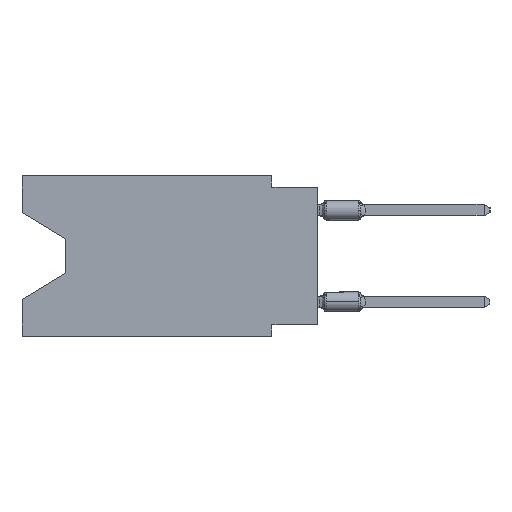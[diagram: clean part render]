
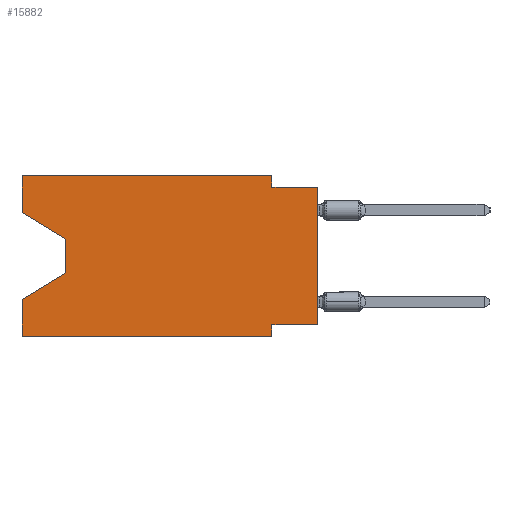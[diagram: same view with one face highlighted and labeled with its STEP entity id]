
A CAD part, left-side view. The second image highlights one B-rep face of the part: STEP entity #15882.
In plain terms, the highlighted planar face has unit normal (-1, 0, 0).
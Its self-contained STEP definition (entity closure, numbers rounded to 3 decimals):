
#258 = VERTEX_POINT ( 'NONE', #11787 ) ;
#295 = CARTESIAN_POINT ( 'NONE',  ( 0., 16.383, 0. ) ) ;
#421 = ORIENTED_EDGE ( 'NONE', *, *, #10246, .F. ) ;
#449 = DIRECTION ( 'NONE',  ( 0., 0., 1. ) ) ;
#477 = VECTOR ( 'NONE', #29039, 1000. ) ;
#811 = VERTEX_POINT ( 'NONE', #11606 ) ;
#919 = VERTEX_POINT ( 'NONE', #9979 ) ;
#1037 = CARTESIAN_POINT ( 'NONE',  ( 0., 13.97, -3.505 ) ) ;
#1049 = VECTOR ( 'NONE', #26966, 1000. ) ;
#1107 = DIRECTION ( 'NONE',  ( 0., 1., 0. ) ) ;
#1323 = VERTEX_POINT ( 'NONE', #10096 ) ;
#1405 = CARTESIAN_POINT ( 'NONE',  ( 0., 16.383, -2.038 ) ) ;
#1774 = LINE ( 'NONE', #10872, #17220 ) ;
#1942 = LINE ( 'NONE', #20669, #10869 ) ;
#2141 = DIRECTION ( 'NONE',  ( 0., 0., -1. ) ) ;
#2292 = LINE ( 'NONE', #16287, #26268 ) ;
#2627 = ORIENTED_EDGE ( 'NONE', *, *, #11034, .F. ) ;
#3143 = DIRECTION ( 'NONE',  ( 0., 0., -1. ) ) ;
#3169 = CARTESIAN_POINT ( 'NONE',  ( 0., 16.383, 0. ) ) ;
#3253 = EDGE_CURVE ( 'NONE', #1323, #10545, #4941, .T. ) ;
#3548 = VERTEX_POINT ( 'NONE', #3169 ) ;
#3642 = CARTESIAN_POINT ( 'NONE',  ( 0., 16.383, -6.852 ) ) ;
#3846 = AXIS2_PLACEMENT_3D ( 'NONE', #5062, #14456, #3143 ) ;
#3945 = VERTEX_POINT ( 'NONE', #5924 ) ;
#4104 = EDGE_CURVE ( 'NONE', #21674, #27669, #26607, .T. ) ;
#4353 = CARTESIAN_POINT ( 'NONE',  ( 0., 2.54, -0.635 ) ) ;
#4443 = DIRECTION ( 'NONE',  ( 0., 0., -1. ) ) ;
#4531 = LINE ( 'NONE', #22835, #7542 ) ;
#4649 = DIRECTION ( 'NONE',  ( 0., 0., 1. ) ) ;
#4802 = CARTESIAN_POINT ( 'NONE',  ( 0., 0., 0. ) ) ;
#4941 = LINE ( 'NONE', #4802, #22387 ) ;
#5062 = CARTESIAN_POINT ( 'NONE',  ( 0., 16.383, 0. ) ) ;
#5570 = CARTESIAN_POINT ( 'NONE',  ( 0., 0., -8.255 ) ) ;
#5795 = ORIENTED_EDGE ( 'NONE', *, *, #9976, .F. ) ;
#5924 = CARTESIAN_POINT ( 'NONE',  ( 0., 2.54, 0. ) ) ;
#6217 = DIRECTION ( 'NONE',  ( 0., 0.855, -0.519 ) ) ;
#6565 = ORIENTED_EDGE ( 'NONE', *, *, #16630, .F. ) ;
#7277 = EDGE_CURVE ( 'NONE', #25201, #27669, #26378, .T. ) ;
#7542 = VECTOR ( 'NONE', #9296, 1000. ) ;
#7638 = EDGE_CURVE ( 'NONE', #258, #21674, #21414, .T. ) ;
#7674 = CARTESIAN_POINT ( 'NONE',  ( 0., 0., -0.635 ) ) ;
#8165 = VECTOR ( 'NONE', #16582, 1000. ) ;
#8186 = ORIENTED_EDGE ( 'NONE', *, *, #14521, .F. ) ;
#9095 = DIRECTION ( 'NONE',  ( 0., -0.855, -0.519 ) ) ;
#9296 = DIRECTION ( 'NONE',  ( 0., -1., 0. ) ) ;
#9976 = EDGE_CURVE ( 'NONE', #11343, #10545, #21335, .T. ) ;
#9979 = CARTESIAN_POINT ( 'NONE',  ( 0., 2.54, -8.89 ) ) ;
#10014 = EDGE_CURVE ( 'NONE', #1323, #811, #25963, .T. ) ;
#10096 = CARTESIAN_POINT ( 'NONE',  ( 0., 0., -8.255 ) ) ;
#10246 = EDGE_CURVE ( 'NONE', #3548, #3945, #22795, .T. ) ;
#10502 = CARTESIAN_POINT ( 'NONE',  ( 0., 13.97, -5.385 ) ) ;
#10545 = VERTEX_POINT ( 'NONE', #11131 ) ;
#10691 = CARTESIAN_POINT ( 'NONE',  ( 0., 13.97, -5.385 ) ) ;
#10869 = VECTOR ( 'NONE', #9095, 1000. ) ;
#10872 = CARTESIAN_POINT ( 'NONE',  ( 0., 2.54, -8.89 ) ) ;
#10891 = ORIENTED_EDGE ( 'NONE', *, *, #7638, .T. ) ;
#11034 = EDGE_CURVE ( 'NONE', #3945, #11343, #2292, .T. ) ;
#11131 = CARTESIAN_POINT ( 'NONE',  ( 0., 0., -0.635 ) ) ;
#11343 = VERTEX_POINT ( 'NONE', #4353 ) ;
#11345 = CARTESIAN_POINT ( 'NONE',  ( 0., 16.383, 0. ) ) ;
#11606 = CARTESIAN_POINT ( 'NONE',  ( 0., 2.54, -8.255 ) ) ;
#11661 = ORIENTED_EDGE ( 'NONE', *, *, #7277, .F. ) ;
#11787 = CARTESIAN_POINT ( 'NONE',  ( 0., 13.97, -3.505 ) ) ;
#14327 = CARTESIAN_POINT ( 'NONE',  ( 0., 16.383, -8.89 ) ) ;
#14456 = DIRECTION ( 'NONE',  ( 1., 0., 0. ) ) ;
#14521 = EDGE_CURVE ( 'NONE', #811, #919, #1774, .T. ) ;
#14915 = CARTESIAN_POINT ( 'NONE',  ( 0., 16.383, 0. ) ) ;
#15882 = ADVANCED_FACE ( 'NONE', ( #25921 ), #23684, .F. ) ;
#16287 = CARTESIAN_POINT ( 'NONE',  ( 0., 2.54, 0. ) ) ;
#16582 = DIRECTION ( 'NONE',  ( 0., -1., 0. ) ) ;
#16630 = EDGE_CURVE ( 'NONE', #21735, #3548, #18450, .T. ) ;
#17220 = VECTOR ( 'NONE', #4443, 1000. ) ;
#17449 = VECTOR ( 'NONE', #6217, 1000. ) ;
#18430 = DIRECTION ( 'NONE',  ( 0., 0., -1. ) ) ;
#18450 = LINE ( 'NONE', #295, #26042 ) ;
#18553 = VECTOR ( 'NONE', #18430, 1000. ) ;
#20669 = CARTESIAN_POINT ( 'NONE',  ( 0., 16.383, -2.038 ) ) ;
#21335 = LINE ( 'NONE', #7674, #8165 ) ;
#21414 = LINE ( 'NONE', #1037, #18553 ) ;
#21674 = VERTEX_POINT ( 'NONE', #10502 ) ;
#21735 = VERTEX_POINT ( 'NONE', #1405 ) ;
#22387 = VECTOR ( 'NONE', #4649, 1000. ) ;
#22389 = VECTOR ( 'NONE', #1107, 1000. ) ;
#22662 = ORIENTED_EDGE ( 'NONE', *, *, #27413, .T. ) ;
#22795 = LINE ( 'NONE', #11345, #1049 ) ;
#22835 = CARTESIAN_POINT ( 'NONE',  ( 0., 16.383, -8.89 ) ) ;
#22997 = ORIENTED_EDGE ( 'NONE', *, *, #4104, .T. ) ;
#23684 = PLANE ( 'NONE',  #3846 ) ;
#24524 = ORIENTED_EDGE ( 'NONE', *, *, #10014, .F. ) ;
#25201 = VERTEX_POINT ( 'NONE', #14327 ) ;
#25460 = EDGE_CURVE ( 'NONE', #21735, #258, #1942, .T. ) ;
#25921 = FACE_OUTER_BOUND ( 'NONE', #29209, .T. ) ;
#25963 = LINE ( 'NONE', #5570, #22389 ) ;
#26042 = VECTOR ( 'NONE', #449, 1000. ) ;
#26268 = VECTOR ( 'NONE', #2141, 1000. ) ;
#26378 = LINE ( 'NONE', #14915, #477 ) ;
#26607 = LINE ( 'NONE', #10691, #17449 ) ;
#26966 = DIRECTION ( 'NONE',  ( 0., -1., 0. ) ) ;
#27293 = ORIENTED_EDGE ( 'NONE', *, *, #25460, .T. ) ;
#27413 = EDGE_CURVE ( 'NONE', #25201, #919, #4531, .T. ) ;
#27669 = VERTEX_POINT ( 'NONE', #3642 ) ;
#28668 = ORIENTED_EDGE ( 'NONE', *, *, #3253, .T. ) ;
#29039 = DIRECTION ( 'NONE',  ( 0., 0., 1. ) ) ;
#29209 = EDGE_LOOP ( 'NONE', ( #27293, #10891, #22997, #11661, #22662, #8186, #24524, #28668, #5795, #2627, #421, #6565 ) ) ;
